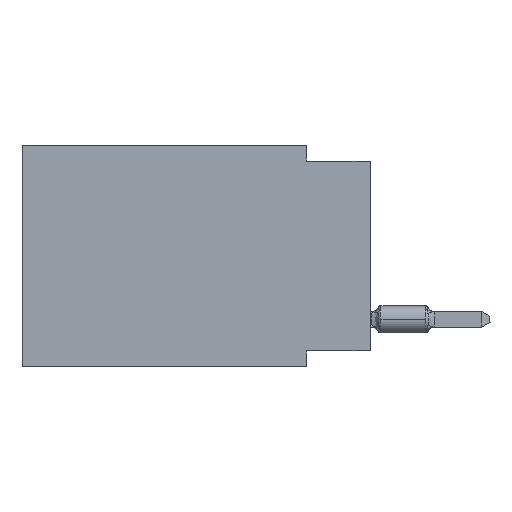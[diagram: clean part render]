
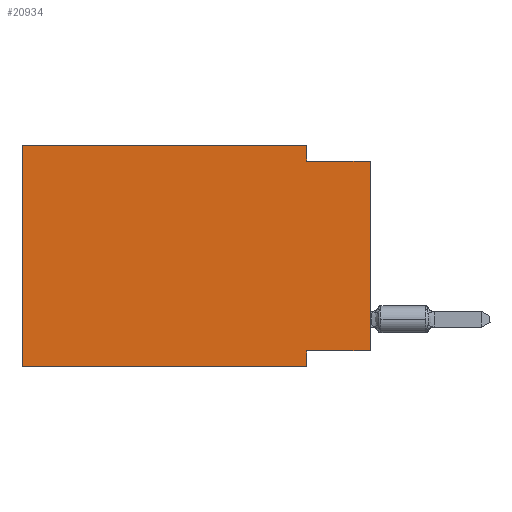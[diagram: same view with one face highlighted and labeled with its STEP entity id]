
A CAD part, left-side view. The second image highlights one B-rep face of the part: STEP entity #20934.
In plain terms, the highlighted planar face has unit normal (-1, 0, 0).
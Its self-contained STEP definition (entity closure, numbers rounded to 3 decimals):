
#45 = ORIENTED_EDGE ( 'NONE', *, *, #7337, .F. ) ;
#242 = DIRECTION ( 'NONE',  ( 0., 0., -1. ) ) ;
#600 = CARTESIAN_POINT ( 'NONE',  ( 0., 13.97, 0. ) ) ;
#737 = LINE ( 'NONE', #21481, #16518 ) ;
#887 = CARTESIAN_POINT ( 'NONE',  ( 0., 2.54, -8.89 ) ) ;
#1466 = CARTESIAN_POINT ( 'NONE',  ( 0., 2.54, -8.89 ) ) ;
#1721 = EDGE_CURVE ( 'NONE', #12483, #23308, #19669, .T. ) ;
#2168 = CARTESIAN_POINT ( 'NONE',  ( 0., 0., -8.255 ) ) ;
#2184 = LINE ( 'NONE', #8869, #20194 ) ;
#2304 = EDGE_CURVE ( 'NONE', #11385, #10311, #23547, .T. ) ;
#2716 = DIRECTION ( 'NONE',  ( 0., -1., 0. ) ) ;
#3947 = PLANE ( 'NONE',  #6373 ) ;
#4407 = EDGE_CURVE ( 'NONE', #23308, #11385, #9684, .T. ) ;
#5781 = EDGE_CURVE ( 'NONE', #11002, #20630, #18291, .T. ) ;
#6192 = CARTESIAN_POINT ( 'NONE',  ( 0., 2.54, -0.635 ) ) ;
#6373 = AXIS2_PLACEMENT_3D ( 'NONE', #9592, #7868, #242 ) ;
#6575 = ORIENTED_EDGE ( 'NONE', *, *, #8938, .T. ) ;
#6646 = LINE ( 'NONE', #10566, #19479 ) ;
#6677 = ORIENTED_EDGE ( 'NONE', *, *, #4407, .F. ) ;
#7337 = EDGE_CURVE ( 'NONE', #20295, #12483, #23282, .T. ) ;
#7868 = DIRECTION ( 'NONE',  ( 1., 0., 0. ) ) ;
#7987 = DIRECTION ( 'NONE',  ( 0., 0., 1. ) ) ;
#8659 = ORIENTED_EDGE ( 'NONE', *, *, #10414, .F. ) ;
#8789 = VECTOR ( 'NONE', #15966, 1000. ) ;
#8869 = CARTESIAN_POINT ( 'NONE',  ( 0., 0., -8.255 ) ) ;
#8938 = EDGE_CURVE ( 'NONE', #13519, #10311, #737, .T. ) ;
#9592 = CARTESIAN_POINT ( 'NONE',  ( 0., 13.97, 0. ) ) ;
#9618 = CARTESIAN_POINT ( 'NONE',  ( 0., 2.54, 0. ) ) ;
#9684 = LINE ( 'NONE', #15197, #23720 ) ;
#9791 = ORIENTED_EDGE ( 'NONE', *, *, #2304, .F. ) ;
#10277 = ORIENTED_EDGE ( 'NONE', *, *, #1721, .F. ) ;
#10311 = VERTEX_POINT ( 'NONE', #17173 ) ;
#10414 = EDGE_CURVE ( 'NONE', #13519, #11002, #2184, .T. ) ;
#10566 = CARTESIAN_POINT ( 'NONE',  ( 0., 13.97, -8.89 ) ) ;
#10896 = VECTOR ( 'NONE', #16081, 1000. ) ;
#11002 = VERTEX_POINT ( 'NONE', #11866 ) ;
#11385 = VERTEX_POINT ( 'NONE', #6192 ) ;
#11866 = CARTESIAN_POINT ( 'NONE',  ( 0., 2.54, -8.255 ) ) ;
#12483 = VERTEX_POINT ( 'NONE', #18453 ) ;
#13493 = DIRECTION ( 'NONE',  ( 0., 0., -1. ) ) ;
#13519 = VERTEX_POINT ( 'NONE', #2168 ) ;
#14624 = VECTOR ( 'NONE', #2716, 1000. ) ;
#15197 = CARTESIAN_POINT ( 'NONE',  ( 0., 2.54, 0. ) ) ;
#15966 = DIRECTION ( 'NONE',  ( 0., -1., 0. ) ) ;
#16081 = DIRECTION ( 'NONE',  ( 0., 0., -1. ) ) ;
#16351 = DIRECTION ( 'NONE',  ( 0., 1., 0. ) ) ;
#16518 = VECTOR ( 'NONE', #7987, 1000. ) ;
#17173 = CARTESIAN_POINT ( 'NONE',  ( 0., 0., -0.635 ) ) ;
#17822 = CARTESIAN_POINT ( 'NONE',  ( 0., 13.97, 0. ) ) ;
#17867 = CARTESIAN_POINT ( 'NONE',  ( 0., 13.97, -8.89 ) ) ;
#18291 = LINE ( 'NONE', #1466, #10896 ) ;
#18453 = CARTESIAN_POINT ( 'NONE',  ( 0., 13.97, 0. ) ) ;
#18806 = FACE_OUTER_BOUND ( 'NONE', #21859, .T. ) ;
#18825 = ORIENTED_EDGE ( 'NONE', *, *, #22359, .T. ) ;
#19479 = VECTOR ( 'NONE', #19546, 1000. ) ;
#19546 = DIRECTION ( 'NONE',  ( 0., -1., 0. ) ) ;
#19547 = CARTESIAN_POINT ( 'NONE',  ( 0., 0., -0.635 ) ) ;
#19669 = LINE ( 'NONE', #17822, #8789 ) ;
#20194 = VECTOR ( 'NONE', #16351, 1000. ) ;
#20295 = VERTEX_POINT ( 'NONE', #17867 ) ;
#20393 = VECTOR ( 'NONE', #21112, 1000. ) ;
#20630 = VERTEX_POINT ( 'NONE', #887 ) ;
#20934 = ADVANCED_FACE ( 'NONE', ( #18806 ), #3947, .F. ) ;
#21112 = DIRECTION ( 'NONE',  ( 0., 0., 1. ) ) ;
#21481 = CARTESIAN_POINT ( 'NONE',  ( 0., 0., 0. ) ) ;
#21645 = ORIENTED_EDGE ( 'NONE', *, *, #5781, .F. ) ;
#21859 = EDGE_LOOP ( 'NONE', ( #6575, #9791, #6677, #10277, #45, #18825, #21645, #8659 ) ) ;
#22359 = EDGE_CURVE ( 'NONE', #20295, #20630, #6646, .T. ) ;
#23282 = LINE ( 'NONE', #600, #20393 ) ;
#23308 = VERTEX_POINT ( 'NONE', #9618 ) ;
#23547 = LINE ( 'NONE', #19547, #14624 ) ;
#23720 = VECTOR ( 'NONE', #13493, 1000. ) ;
